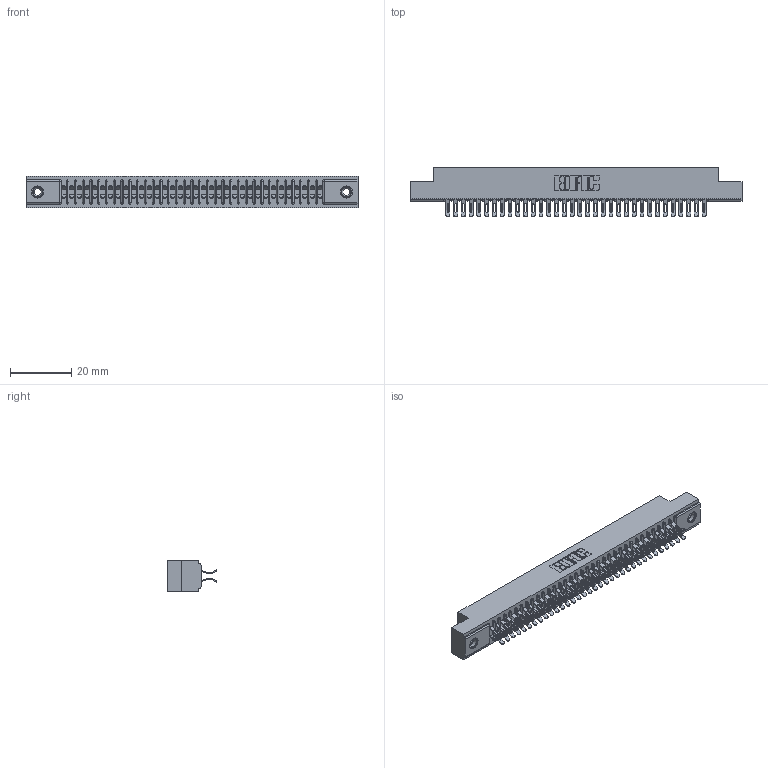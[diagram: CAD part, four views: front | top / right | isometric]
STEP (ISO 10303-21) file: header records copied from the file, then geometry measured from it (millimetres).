
FILE_DESCRIPTION (( 'STEP AP203' ), '1' );
FILE_NAME ('341-068-555-208.STEP', '2018-08-07T19:13:27', ( '' ), ( '' ), 'SwSTEP 2.0', 'SolidWorks 2016', '' );
FILE_SCHEMA (( 'CONFIG_CONTROL_DESIGN' ));
Length unit declared in the file: inch
Products named in the file (4): 341 Part_.156 (3.96) Dia Mounting Holes; 341-292-001_341-292-155; 345-250-001_345-250-003-102; 341-068-555-208
Assembly tree (71 placements, depth 2):
  341-068-555-208
    341 Part_.156 (3.96) Dia Mounting Holes
    341-292-001_341-292-155  x68
    345-250-001_345-250-003-102  x2
Bounding box: 108.58 x 16.31 x 10.16 mm (x, y, z)
Volume: 8091.3 mm3; surface area: 14684.2 mm2
Topology: 71 solids, 71 shells, 5480 faces, 16330 edges, 10626 vertices
Faces by surface type: plane 2956, cylinder 2372, sphere 70, torus 70, cone 12
Entity records: 43868 total; most frequent: CARTESIAN_POINT 7291, ORIENTED_EDGE 7228, DIRECTION 7082, EDGE_CURVE 3614, LINE 2892, VECTOR 2892, VERTEX_POINT 2288, AXIS2_PLACEMENT_3D 2095
